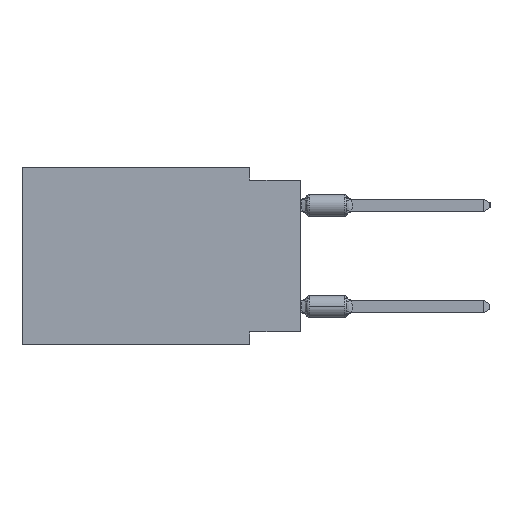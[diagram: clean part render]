
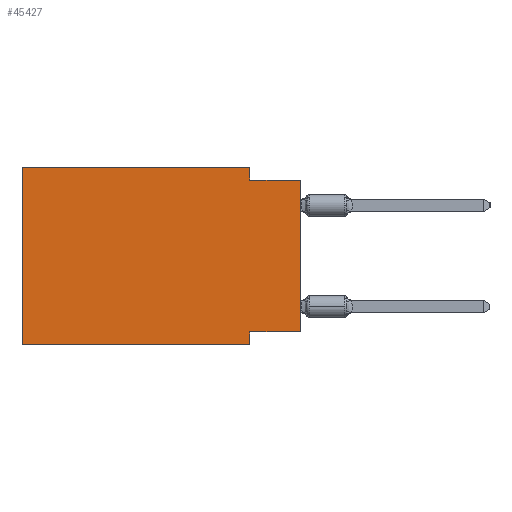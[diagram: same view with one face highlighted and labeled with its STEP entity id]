
A CAD part, left-side view. The second image highlights one B-rep face of the part: STEP entity #45427.
In plain terms, the highlighted planar face has unit normal (-1, 0, 0).
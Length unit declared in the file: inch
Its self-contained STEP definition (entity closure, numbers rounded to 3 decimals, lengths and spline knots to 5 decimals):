
#506 = ORIENTED_EDGE ( 'NONE', *, *, #19081, .F. ) ;
#884 = CARTESIAN_POINT ( 'NONE',  ( 0., 0.55, -0.35 ) ) ;
#1062 = DIRECTION ( 'NONE',  ( 0., -1., 0. ) ) ;
#1095 = VECTOR ( 'NONE', #1062, 39.37008 ) ;
#1509 = DIRECTION ( 'NONE',  ( 0., -1., 0. ) ) ;
#3001 = CARTESIAN_POINT ( 'NONE',  ( 0., 0.1, -0.325 ) ) ;
#3649 = EDGE_CURVE ( 'NONE', #38253, #30740, #38610, .T. ) ;
#4999 = LINE ( 'NONE', #21899, #42621 ) ;
#6661 = LINE ( 'NONE', #23019, #12077 ) ;
#7214 = EDGE_CURVE ( 'NONE', #22780, #30740, #4999, .T. ) ;
#7363 = VERTEX_POINT ( 'NONE', #51992 ) ;
#8970 = VECTOR ( 'NONE', #30451, 39.37008 ) ;
#9091 = LINE ( 'NONE', #13904, #1095 ) ;
#10850 = ORIENTED_EDGE ( 'NONE', *, *, #20184, .F. ) ;
#11129 = ORIENTED_EDGE ( 'NONE', *, *, #7214, .T. ) ;
#11659 = FACE_OUTER_BOUND ( 'NONE', #15212, .T. ) ;
#12077 = VECTOR ( 'NONE', #47754, 39.37008 ) ;
#12197 = ORIENTED_EDGE ( 'NONE', *, *, #3649, .F. ) ;
#12262 = CARTESIAN_POINT ( 'NONE',  ( 0., 0., -0.325 ) ) ;
#12470 = CARTESIAN_POINT ( 'NONE',  ( 0., 0.1, -0.025 ) ) ;
#13028 = VECTOR ( 'NONE', #35079, 39.37008 ) ;
#13904 = CARTESIAN_POINT ( 'NONE',  ( 0., 0.55, 0. ) ) ;
#15212 = EDGE_LOOP ( 'NONE', ( #39329, #506, #16573, #10850, #45687, #11129, #12197, #39453 ) ) ;
#15232 = VERTEX_POINT ( 'NONE', #40800 ) ;
#15642 = EDGE_CURVE ( 'NONE', #21938, #38253, #36705, .T. ) ;
#15946 = PLANE ( 'NONE',  #21049 ) ;
#16573 = ORIENTED_EDGE ( 'NONE', *, *, #39056, .F. ) ;
#17915 = DIRECTION ( 'NONE',  ( 0., 0., -1. ) ) ;
#18901 = LINE ( 'NONE', #38790, #8970 ) ;
#19081 = EDGE_CURVE ( 'NONE', #27476, #30517, #18901, .T. ) ;
#19725 = CARTESIAN_POINT ( 'NONE',  ( 0., 0.55, 0. ) ) ;
#20184 = EDGE_CURVE ( 'NONE', #7363, #15232, #9091, .T. ) ;
#21049 = AXIS2_PLACEMENT_3D ( 'NONE', #19725, #39877, #31540 ) ;
#21648 = CARTESIAN_POINT ( 'NONE',  ( 0., 0., -0.325 ) ) ;
#21899 = CARTESIAN_POINT ( 'NONE',  ( 0., 0.55, -0.35 ) ) ;
#21938 = VERTEX_POINT ( 'NONE', #21648 ) ;
#22579 = VECTOR ( 'NONE', #51639, 39.37008 ) ;
#22780 = VERTEX_POINT ( 'NONE', #884 ) ;
#23019 = CARTESIAN_POINT ( 'NONE',  ( 0., 0., 0. ) ) ;
#24334 = DIRECTION ( 'NONE',  ( 0., 1., 0. ) ) ;
#26279 = CARTESIAN_POINT ( 'NONE',  ( 0., 0.1, -0.35 ) ) ;
#26487 = CARTESIAN_POINT ( 'NONE',  ( 0., 0.1, -0.35 ) ) ;
#26743 = LINE ( 'NONE', #50938, #13028 ) ;
#27476 = VERTEX_POINT ( 'NONE', #12470 ) ;
#30451 = DIRECTION ( 'NONE',  ( 0., -1., 0. ) ) ;
#30517 = VERTEX_POINT ( 'NONE', #30645 ) ;
#30645 = CARTESIAN_POINT ( 'NONE',  ( 0., 0., -0.025 ) ) ;
#30740 = VERTEX_POINT ( 'NONE', #26279 ) ;
#31020 = VECTOR ( 'NONE', #24334, 39.37008 ) ;
#31540 = DIRECTION ( 'NONE',  ( 0., 0., -1. ) ) ;
#35079 = DIRECTION ( 'NONE',  ( 0., 0., -1. ) ) ;
#35674 = EDGE_CURVE ( 'NONE', #21938, #30517, #6661, .T. ) ;
#36705 = LINE ( 'NONE', #12262, #31020 ) ;
#38253 = VERTEX_POINT ( 'NONE', #3001 ) ;
#38610 = LINE ( 'NONE', #26487, #47358 ) ;
#38790 = CARTESIAN_POINT ( 'NONE',  ( 0., 0., -0.025 ) ) ;
#39056 = EDGE_CURVE ( 'NONE', #15232, #27476, #26743, .T. ) ;
#39329 = ORIENTED_EDGE ( 'NONE', *, *, #35674, .T. ) ;
#39453 = ORIENTED_EDGE ( 'NONE', *, *, #15642, .F. ) ;
#39877 = DIRECTION ( 'NONE',  ( 1., 0., 0. ) ) ;
#40800 = CARTESIAN_POINT ( 'NONE',  ( 0., 0.1, 0. ) ) ;
#42469 = EDGE_CURVE ( 'NONE', #22780, #7363, #50833, .T. ) ;
#42621 = VECTOR ( 'NONE', #1509, 39.37008 ) ;
#45427 = ADVANCED_FACE ( 'NONE', ( #11659 ), #15946, .F. ) ;
#45687 = ORIENTED_EDGE ( 'NONE', *, *, #42469, .F. ) ;
#47358 = VECTOR ( 'NONE', #17915, 39.37008 ) ;
#47754 = DIRECTION ( 'NONE',  ( 0., 0., 1. ) ) ;
#50833 = LINE ( 'NONE', #51092, #22579 ) ;
#50938 = CARTESIAN_POINT ( 'NONE',  ( 0., 0.1, 0. ) ) ;
#51092 = CARTESIAN_POINT ( 'NONE',  ( 0., 0.55, 0. ) ) ;
#51639 = DIRECTION ( 'NONE',  ( 0., 0., 1. ) ) ;
#51992 = CARTESIAN_POINT ( 'NONE',  ( 0., 0.55, 0. ) ) ;
